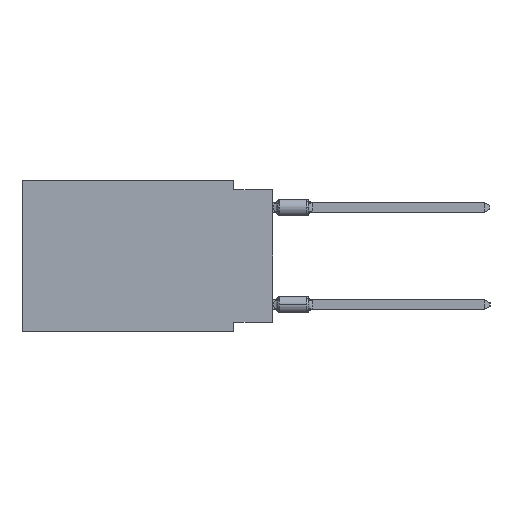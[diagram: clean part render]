
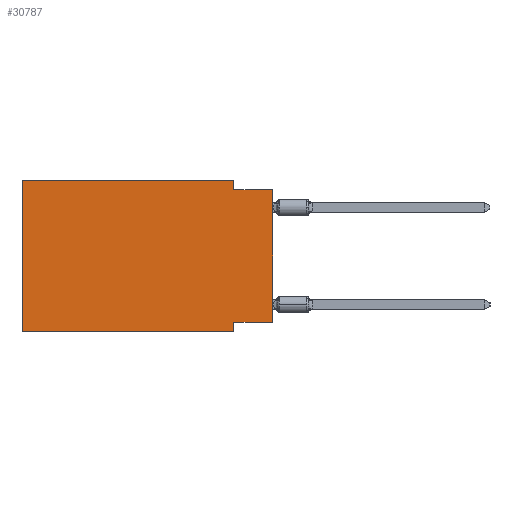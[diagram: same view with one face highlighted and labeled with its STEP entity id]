
A CAD part, left-side view. The second image highlights one B-rep face of the part: STEP entity #30787.
In plain terms, the highlighted planar face has unit normal (-1, 0, 0).
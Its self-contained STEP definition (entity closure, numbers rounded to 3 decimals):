
#1265 = CARTESIAN_POINT ( 'NONE',  ( 0., 16.383, -9.906 ) ) ;
#1436 = LINE ( 'NONE', #14528, #17425 ) ;
#1616 = LINE ( 'NONE', #19850, #16979 ) ;
#2271 = CARTESIAN_POINT ( 'NONE',  ( 0., 2.54, 0. ) ) ;
#3696 = CARTESIAN_POINT ( 'NONE',  ( 0., 2.54, -9.906 ) ) ;
#4578 = EDGE_CURVE ( 'NONE', #32891, #23114, #38541, .T. ) ;
#4607 = VECTOR ( 'NONE', #37792, 1000. ) ;
#5971 = EDGE_CURVE ( 'NONE', #20670, #42428, #29157, .T. ) ;
#10145 = LINE ( 'NONE', #56077, #24143 ) ;
#10425 = VECTOR ( 'NONE', #46826, 1000. ) ;
#11180 = CARTESIAN_POINT ( 'NONE',  ( 0., 0., -9.271 ) ) ;
#11799 = ORIENTED_EDGE ( 'NONE', *, *, #46371, .T. ) ;
#11839 = CARTESIAN_POINT ( 'NONE',  ( 0., 16.383, 0. ) ) ;
#14359 = VERTEX_POINT ( 'NONE', #3696 ) ;
#14528 = CARTESIAN_POINT ( 'NONE',  ( 0., 16.383, 0. ) ) ;
#14884 = LINE ( 'NONE', #32311, #52029 ) ;
#15503 = PLANE ( 'NONE',  #38277 ) ;
#15782 = FACE_OUTER_BOUND ( 'NONE', #30096, .T. ) ;
#16273 = VERTEX_POINT ( 'NONE', #11839 ) ;
#16979 = VECTOR ( 'NONE', #37535, 1000. ) ;
#17076 = CARTESIAN_POINT ( 'NONE',  ( 0., 0., -0.635 ) ) ;
#17425 = VECTOR ( 'NONE', #36235, 1000. ) ;
#18605 = DIRECTION ( 'NONE',  ( 0., 0., -1. ) ) ;
#19792 = DIRECTION ( 'NONE',  ( 0., 0., -1. ) ) ;
#19850 = CARTESIAN_POINT ( 'NONE',  ( 0., 16.383, -9.906 ) ) ;
#20670 = VERTEX_POINT ( 'NONE', #52305 ) ;
#21290 = ORIENTED_EDGE ( 'NONE', *, *, #47250, .F. ) ;
#22667 = VERTEX_POINT ( 'NONE', #17076 ) ;
#23114 = VERTEX_POINT ( 'NONE', #47202 ) ;
#24143 = VECTOR ( 'NONE', #50657, 1000. ) ;
#25454 = ORIENTED_EDGE ( 'NONE', *, *, #4578, .F. ) ;
#26630 = DIRECTION ( 'NONE',  ( 0., 0., 1. ) ) ;
#29157 = LINE ( 'NONE', #11180, #55224 ) ;
#29217 = LINE ( 'NONE', #54917, #4607 ) ;
#30096 = EDGE_LOOP ( 'NONE', ( #11799, #43641, #25454, #21290, #41343, #35109, #44729, #48855 ) ) ;
#30787 = ADVANCED_FACE ( 'NONE', ( #15782 ), #15503, .F. ) ;
#32311 = CARTESIAN_POINT ( 'NONE',  ( 0., 2.54, -9.906 ) ) ;
#32637 = CARTESIAN_POINT ( 'NONE',  ( 0., 16.383, 0. ) ) ;
#32891 = VERTEX_POINT ( 'NONE', #2271 ) ;
#35109 = ORIENTED_EDGE ( 'NONE', *, *, #40698, .T. ) ;
#36235 = DIRECTION ( 'NONE',  ( 0., -1., 0. ) ) ;
#37442 = DIRECTION ( 'NONE',  ( 0., 1., 0. ) ) ;
#37535 = DIRECTION ( 'NONE',  ( 0., -1., 0. ) ) ;
#37792 = DIRECTION ( 'NONE',  ( 0., 0., 1. ) ) ;
#38277 = AXIS2_PLACEMENT_3D ( 'NONE', #32637, #42344, #19792 ) ;
#38541 = LINE ( 'NONE', #55673, #10425 ) ;
#39495 = CARTESIAN_POINT ( 'NONE',  ( 0., 16.383, 0. ) ) ;
#40698 = EDGE_CURVE ( 'NONE', #55920, #14359, #1616, .T. ) ;
#41343 = ORIENTED_EDGE ( 'NONE', *, *, #53528, .F. ) ;
#42344 = DIRECTION ( 'NONE',  ( 1., 0., 0. ) ) ;
#42428 = VERTEX_POINT ( 'NONE', #46044 ) ;
#43303 = VECTOR ( 'NONE', #26630, 1000. ) ;
#43641 = ORIENTED_EDGE ( 'NONE', *, *, #53321, .F. ) ;
#44729 = ORIENTED_EDGE ( 'NONE', *, *, #46735, .F. ) ;
#46044 = CARTESIAN_POINT ( 'NONE',  ( 0., 2.54, -9.271 ) ) ;
#46371 = EDGE_CURVE ( 'NONE', #20670, #22667, #29217, .T. ) ;
#46735 = EDGE_CURVE ( 'NONE', #42428, #14359, #14884, .T. ) ;
#46826 = DIRECTION ( 'NONE',  ( 0., 0., -1. ) ) ;
#47202 = CARTESIAN_POINT ( 'NONE',  ( 0., 2.54, -0.635 ) ) ;
#47250 = EDGE_CURVE ( 'NONE', #16273, #32891, #1436, .T. ) ;
#48609 = LINE ( 'NONE', #39495, #43303 ) ;
#48855 = ORIENTED_EDGE ( 'NONE', *, *, #5971, .F. ) ;
#50657 = DIRECTION ( 'NONE',  ( 0., -1., 0. ) ) ;
#52029 = VECTOR ( 'NONE', #18605, 1000. ) ;
#52305 = CARTESIAN_POINT ( 'NONE',  ( 0., 0., -9.271 ) ) ;
#53321 = EDGE_CURVE ( 'NONE', #23114, #22667, #10145, .T. ) ;
#53528 = EDGE_CURVE ( 'NONE', #55920, #16273, #48609, .T. ) ;
#54917 = CARTESIAN_POINT ( 'NONE',  ( 0., 0., 0. ) ) ;
#55224 = VECTOR ( 'NONE', #37442, 1000. ) ;
#55673 = CARTESIAN_POINT ( 'NONE',  ( 0., 2.54, 0. ) ) ;
#55920 = VERTEX_POINT ( 'NONE', #1265 ) ;
#56077 = CARTESIAN_POINT ( 'NONE',  ( 0., 0., -0.635 ) ) ;
